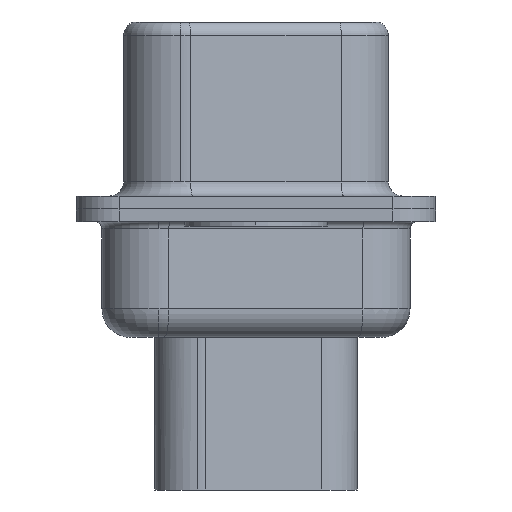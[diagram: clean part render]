
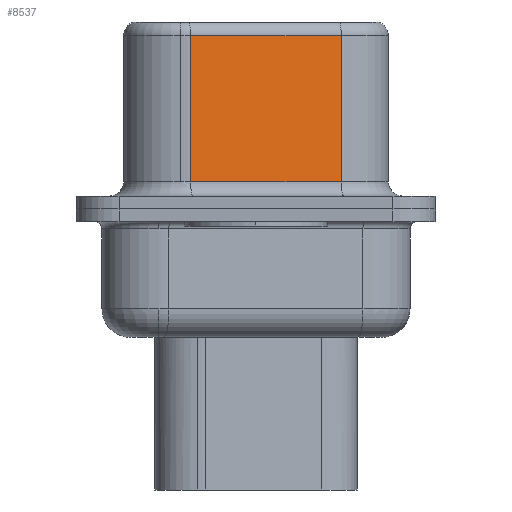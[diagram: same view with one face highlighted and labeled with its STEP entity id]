
A CAD part, left-side view. The second image highlights one B-rep face of the part: STEP entity #8537.
In plain terms, the highlighted planar face has unit normal (-0.985, -0.174, 0).
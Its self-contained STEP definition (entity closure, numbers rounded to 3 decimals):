
#233 = CARTESIAN_POINT ( 'NONE',  ( 4.546, -2.987, 6.07 ) ) ;
#266 = LINE ( 'NONE', #2940, #5572 ) ;
#354 = DIRECTION ( 'NONE',  ( 0.174, -0.985, 0. ) ) ;
#786 = DIRECTION ( 'NONE',  ( -0.174, 0.985, 0. ) ) ;
#874 = ORIENTED_EDGE ( 'NONE', *, *, #1677, .T. ) ;
#900 = ORIENTED_EDGE ( 'NONE', *, *, #10897, .T. ) ;
#1434 = DIRECTION ( 'NONE',  ( 0.985, 0.174, 0. ) ) ;
#1677 = EDGE_CURVE ( 'NONE', #8741, #10858, #1798, .T. ) ;
#1737 = CARTESIAN_POINT ( 'NONE',  ( 3.615, 2.293, 0.95 ) ) ;
#1798 = LINE ( 'NONE', #8933, #9998 ) ;
#1875 = CARTESIAN_POINT ( 'NONE',  ( 3.615, 2.293, 6.57 ) ) ;
#2163 = DIRECTION ( 'NONE',  ( 0., 0., -1. ) ) ;
#2323 = CARTESIAN_POINT ( 'NONE',  ( 4.546, -2.987, 6.57 ) ) ;
#2884 = LINE ( 'NONE', #1875, #5535 ) ;
#2940 = CARTESIAN_POINT ( 'NONE',  ( 4.546, -2.987, 6.57 ) ) ;
#3166 = EDGE_CURVE ( 'NONE', #8741, #10679, #266, .T. ) ;
#4076 = AXIS2_PLACEMENT_3D ( 'NONE', #2323, #1434, #7858 ) ;
#4148 = EDGE_CURVE ( 'NONE', #8186, #10679, #4983, .T. ) ;
#4169 = ORIENTED_EDGE ( 'NONE', *, *, #3166, .F. ) ;
#4228 = FACE_OUTER_BOUND ( 'NONE', #9291, .T. ) ;
#4983 = LINE ( 'NONE', #11295, #5783 ) ;
#5535 = VECTOR ( 'NONE', #5671, 1000. ) ;
#5572 = VECTOR ( 'NONE', #2163, 1000. ) ;
#5671 = DIRECTION ( 'NONE',  ( 0., 0., -1. ) ) ;
#5783 = VECTOR ( 'NONE', #354, 1000. ) ;
#7422 = ORIENTED_EDGE ( 'NONE', *, *, #4148, .T. ) ;
#7738 = PLANE ( 'NONE',  #4076 ) ;
#7858 = DIRECTION ( 'NONE',  ( -0.174, 0.985, 0. ) ) ;
#8186 = VERTEX_POINT ( 'NONE', #1737 ) ;
#8471 = CARTESIAN_POINT ( 'NONE',  ( 3.615, 2.293, 6.07 ) ) ;
#8537 = ADVANCED_FACE ( 'NONE', ( #4228 ), #7738, .F. ) ;
#8741 = VERTEX_POINT ( 'NONE', #233 ) ;
#8933 = CARTESIAN_POINT ( 'NONE',  ( 4.546, -2.987, 6.07 ) ) ;
#9291 = EDGE_LOOP ( 'NONE', ( #4169, #874, #900, #7422 ) ) ;
#9485 = CARTESIAN_POINT ( 'NONE',  ( 4.546, -2.987, 0.95 ) ) ;
#9998 = VECTOR ( 'NONE', #786, 1000. ) ;
#10679 = VERTEX_POINT ( 'NONE', #9485 ) ;
#10858 = VERTEX_POINT ( 'NONE', #8471 ) ;
#10897 = EDGE_CURVE ( 'NONE', #10858, #8186, #2884, .T. ) ;
#11295 = CARTESIAN_POINT ( 'NONE',  ( 4.546, -2.987, 0.95 ) ) ;
